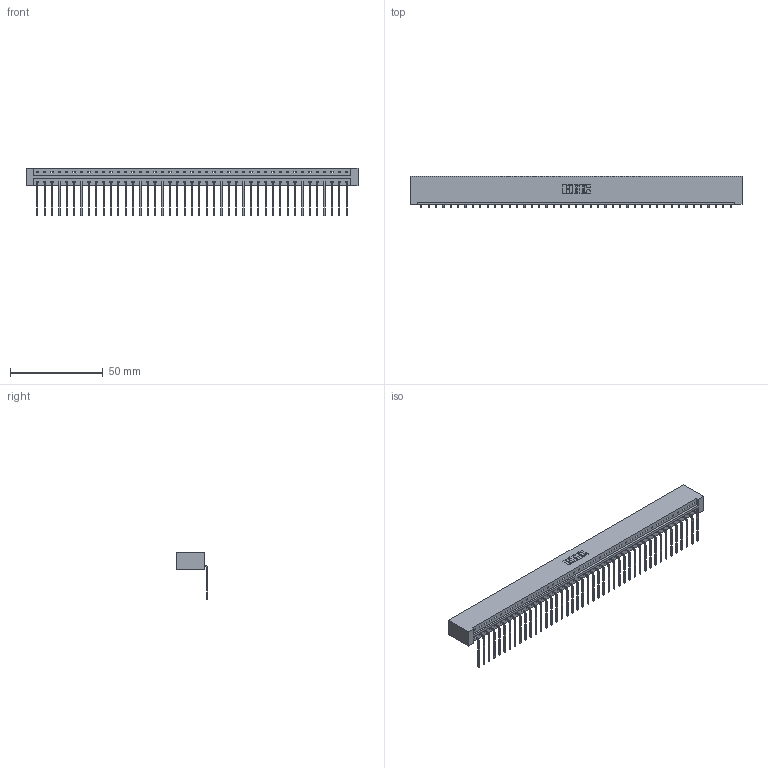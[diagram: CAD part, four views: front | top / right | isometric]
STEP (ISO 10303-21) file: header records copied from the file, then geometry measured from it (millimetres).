
FILE_DESCRIPTION (( 'STEP AP203' ), '1' );
FILE_NAME ('333-043-559-101.STEP', '2018-08-03T20:42:59', ( '' ), ( '' ), 'SwSTEP 2.0', 'SolidWorks 2016', '' );
FILE_SCHEMA (( 'CONFIG_CONTROL_DESIGN' ));
Length unit declared in the file: inch
Products named in the file (3): 345-292-001_558 559 Tail - 1; 333-043-559-101; 333 Part_Lugless
Assembly tree (44 placements, depth 2):
  333-043-559-101
    333 Part_Lugless
    345-292-001_558 559 Tail - 1  x43
Bounding box: 178.64 x 17.09 x 25.53 mm (x, y, z)
Volume: 18740.7 mm3; surface area: 21118.7 mm2
Topology: 44 solids, 44 shells, 2686 faces, 8113 edges, 5350 vertices
Faces by surface type: plane 1958, cylinder 728
Entity records: 25965 total; most frequent: CARTESIAN_POINT 4487, ORIENTED_EDGE 4466, DIRECTION 3775, EDGE_CURVE 2233, LINE 2113, VECTOR 2113, VERTEX_POINT 1486, AXIS2_PLACEMENT_3D 831
